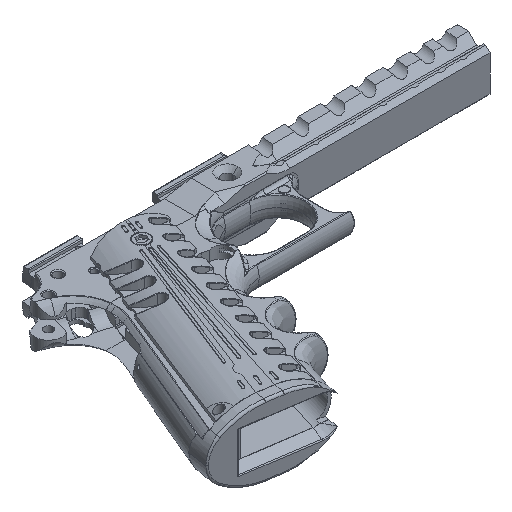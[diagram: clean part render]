
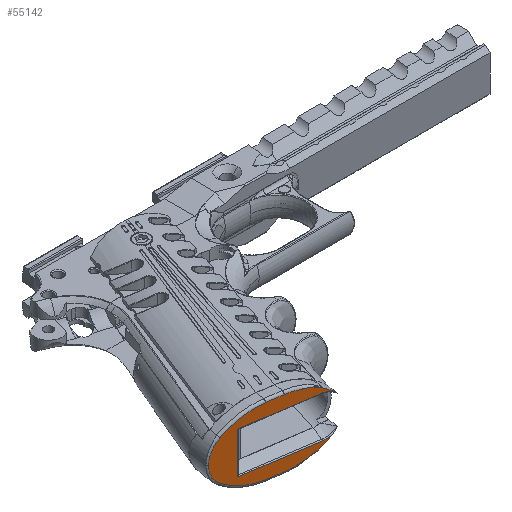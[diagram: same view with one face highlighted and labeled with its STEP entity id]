
A CAD part, isometric view. The second image highlights one B-rep face of the part: STEP entity #55142.
In plain terms, the highlighted face is planar.
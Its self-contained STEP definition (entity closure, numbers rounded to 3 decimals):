
#740 = VERTEX_POINT ( 'NONE', #28184 ) ;
#1054 = VERTEX_POINT ( 'NONE', #53536 ) ;
#1213 = CARTESIAN_POINT ( 'NONE',  ( -13.838, -5.164, 15.002 ) ) ;
#1341 = DIRECTION ( 'NONE',  ( -0.968, 0.25, 0. ) ) ;
#1467 = VERTEX_POINT ( 'NONE', #28141 ) ;
#1565 = DIRECTION ( 'NONE',  ( -0.25, -0.968, 0. ) ) ;
#2685 = AXIS2_PLACEMENT_3D ( 'NONE', #48530, #22746, #52839 ) ;
#5415 = CARTESIAN_POINT ( 'NONE',  ( -35.601, 0.464, -9.336 ) ) ;
#5814 = EDGE_CURVE ( 'NONE', #740, #1467, #17793, .T. ) ;
#6906 = DIRECTION ( 'NONE',  ( -0.25, -0.968, 0. ) ) ;
#7460 = ORIENTED_EDGE ( 'NONE', *, *, #9347, .T. ) ;
#7547 = VERTEX_POINT ( 'NONE', #1213 ) ;
#7964 = CARTESIAN_POINT ( 'NONE',  ( -35.601, 0.464, -9.336 ) ) ;
#8455 = CARTESIAN_POINT ( 'NONE',  ( -21.042, -3.301, -10.872 ) ) ;
#8706 = CARTESIAN_POINT ( 'NONE',  ( -3.333, -7.881, -9.336 ) ) ;
#8812 = CARTESIAN_POINT ( 'NONE',  ( -35.601, 0.464, 0.172 ) ) ;
#8847 = EDGE_LOOP ( 'NONE', ( #16070, #20931, #49724, #31123, #29379, #7460, #43959, #24460, #55542, #18358, #27515, #50691, #26341, #55709, #39166 ) ) ;
#9347 = EDGE_CURVE ( 'NONE', #20665, #36911, #39909, .T. ) ;
#10375 = CARTESIAN_POINT ( 'NONE',  ( -2.664, -8.054, 0. ) ) ;
#10901 = AXIS2_PLACEMENT_3D ( 'NONE', #10375, #40502, #14670 ) ;
#10931 = VERTEX_POINT ( 'NONE', #7964 ) ;
#11095 = CIRCLE ( 'NONE', #32294, 25.874 ) ;
#11402 = EDGE_CURVE ( 'NONE', #1467, #31422, #40404, .T. ) ;
#12796 = DIRECTION ( 'NONE',  ( -0.968, 0.25, 0. ) ) ;
#13134 = EDGE_CURVE ( 'NONE', #34300, #25150, #17911, .T. ) ;
#13143 = DIRECTION ( 'NONE',  ( -0.968, 0.25, 0. ) ) ;
#14338 = CARTESIAN_POINT ( 'NONE',  ( -35.601, 0.464, -0.197 ) ) ;
#14342 = CARTESIAN_POINT ( 'NONE',  ( -26.452, -1.902, -14.417 ) ) ;
#14670 = DIRECTION ( 'NONE',  ( -0.968, 0.25, 0. ) ) ;
#14762 = AXIS2_PLACEMENT_3D ( 'NONE', #15508, #45599, #19800 ) ;
#15508 = CARTESIAN_POINT ( 'NONE',  ( -21.042, -3.301, 10.846 ) ) ;
#15869 = DIRECTION ( 'NONE',  ( 0.968, -0.25, 0. ) ) ;
#16070 = ORIENTED_EDGE ( 'NONE', *, *, #27260, .T. ) ;
#16333 = VERTEX_POINT ( 'NONE', #14342 ) ;
#17274 = LINE ( 'NONE', #41780, #50258 ) ;
#17624 = CIRCLE ( 'NONE', #2685, 24.846 ) ;
#17793 = CIRCLE ( 'NONE', #21756, 9.508 ) ;
#17911 = LINE ( 'NONE', #28651, #39541 ) ;
#18358 = ORIENTED_EDGE ( 'NONE', *, *, #30033, .T. ) ;
#18611 = EDGE_CURVE ( 'NONE', #52695, #1054, #11095, .T. ) ;
#18633 = DIRECTION ( 'NONE',  ( -0.968, 0.25, 0. ) ) ;
#18714 = CARTESIAN_POINT ( 'NONE',  ( 3.48, -9.643, -8.85 ) ) ;
#18730 = CIRCLE ( 'NONE', #35999, 24.846 ) ;
#18989 = VECTOR ( 'NONE', #1341, 1000. ) ;
#19800 = DIRECTION ( 'NONE',  ( -0.968, 0.25, 0. ) ) ;
#20319 = LINE ( 'NONE', #5415, #18989 ) ;
#20665 = VERTEX_POINT ( 'NONE', #47345 ) ;
#20699 = PLANE ( 'NONE',  #49646 ) ;
#20931 = ORIENTED_EDGE ( 'NONE', *, *, #32520, .T. ) ;
#21369 = DIRECTION ( 'NONE',  ( -0.968, 0.25, 0. ) ) ;
#21553 = CARTESIAN_POINT ( 'NONE',  ( -3.616, -7.808, 9.311 ) ) ;
#21756 = AXIS2_PLACEMENT_3D ( 'NONE', #14338, #44456, #18633 ) ;
#22746 = DIRECTION ( 'NONE',  ( -0.25, -0.968, 0. ) ) ;
#24460 = ORIENTED_EDGE ( 'NONE', *, *, #32260, .T. ) ;
#24866 = DIRECTION ( 'NONE',  ( -0.25, -0.968, 0. ) ) ;
#25075 = CARTESIAN_POINT ( 'NONE',  ( -23.833, -2.579, -10.307 ) ) ;
#25150 = VERTEX_POINT ( 'NONE', #34819 ) ;
#25222 = DIRECTION ( 'NONE',  ( -0.968, 0.25, 0. ) ) ;
#25497 = CARTESIAN_POINT ( 'NONE',  ( -14.534, -4.984, 15.002 ) ) ;
#25762 = EDGE_CURVE ( 'NONE', #53487, #20665, #45280, .T. ) ;
#25859 = DIRECTION ( 'NONE',  ( 0.968, -0.25, 0. ) ) ;
#26341 = ORIENTED_EDGE ( 'NONE', *, *, #50733, .T. ) ;
#27244 = CARTESIAN_POINT ( 'NONE',  ( -2.664, -8.054, -0.025 ) ) ;
#27260 = EDGE_CURVE ( 'NONE', #34244, #16333, #17624, .T. ) ;
#27515 = ORIENTED_EDGE ( 'NONE', *, *, #5814, .T. ) ;
#27705 = AXIS2_PLACEMENT_3D ( 'NONE', #27244, #1565, #31617 ) ;
#28141 = CARTESIAN_POINT ( 'NONE',  ( -35.601, 0.464, 9.311 ) ) ;
#28184 = CARTESIAN_POINT ( 'NONE',  ( -39.832, 1.558, 8.247 ) ) ;
#28651 = CARTESIAN_POINT ( 'NONE',  ( -14.534, -4.984, -15.027 ) ) ;
#29379 = ORIENTED_EDGE ( 'NONE', *, *, #25762, .T. ) ;
#29443 = DIRECTION ( 'NONE',  ( 0.968, -0.25, 0. ) ) ;
#30033 = EDGE_CURVE ( 'NONE', #1054, #740, #18730, .T. ) ;
#30694 = CIRCLE ( 'NONE', #14762, 25.874 ) ;
#31123 = ORIENTED_EDGE ( 'NONE', *, *, #46734, .T. ) ;
#31409 = LINE ( 'NONE', #25497, #38819 ) ;
#31422 = VERTEX_POINT ( 'NONE', #47981 ) ;
#31617 = DIRECTION ( 'NONE',  ( -0.968, 0.25, 0. ) ) ;
#32260 = EDGE_CURVE ( 'NONE', #7547, #52695, #31409, .T. ) ;
#32294 = AXIS2_PLACEMENT_3D ( 'NONE', #8455, #38609, #12796 ) ;
#32520 = EDGE_CURVE ( 'NONE', #16333, #34300, #30694, .T. ) ;
#32710 = CARTESIAN_POINT ( 'NONE',  ( -14.534, -4.984, 16.039 ) ) ;
#34244 = VERTEX_POINT ( 'NONE', #53282 ) ;
#34300 = VERTEX_POINT ( 'NONE', #51211 ) ;
#34819 = CARTESIAN_POINT ( 'NONE',  ( -13.838, -5.164, -15.027 ) ) ;
#35051 = EDGE_CURVE ( 'NONE', #39583, #10931, #20319, .T. ) ;
#35999 = AXIS2_PLACEMENT_3D ( 'NONE', #25075, #55162, #29443 ) ;
#36624 = AXIS2_PLACEMENT_3D ( 'NONE', #8812, #38960, #13143 ) ;
#36911 = VERTEX_POINT ( 'NONE', #51225 ) ;
#37058 = DIRECTION ( 'NONE',  ( -0.968, 0.25, 0. ) ) ;
#38108 = CARTESIAN_POINT ( 'NONE',  ( -14.534, -4.984, 16.039 ) ) ;
#38609 = DIRECTION ( 'NONE',  ( -0.25, -0.968, 0. ) ) ;
#38819 = VECTOR ( 'NONE', #21369, 1000. ) ;
#38960 = DIRECTION ( 'NONE',  ( 0.25, 0.968, 0. ) ) ;
#39166 = ORIENTED_EDGE ( 'NONE', *, *, #51722, .T. ) ;
#39541 = VECTOR ( 'NONE', #15869, 1000. ) ;
#39583 = VERTEX_POINT ( 'NONE', #8706 ) ;
#39909 = CIRCLE ( 'NONE', #27705, 10.89 ) ;
#40404 = LINE ( 'NONE', #21553, #51767 ) ;
#40502 = DIRECTION ( 'NONE',  ( -0.25, -0.968, 0. ) ) ;
#41120 = AXIS2_PLACEMENT_3D ( 'NONE', #50655, #24866, #54961 ) ;
#41780 = CARTESIAN_POINT ( 'NONE',  ( -3.333, -7.881, -8.998 ) ) ;
#41970 = DIRECTION ( 'NONE',  ( 0., 0., -1. ) ) ;
#43798 = CIRCLE ( 'NONE', #41120, 31.075 ) ;
#43959 = ORIENTED_EDGE ( 'NONE', *, *, #48716, .T. ) ;
#44456 = DIRECTION ( 'NONE',  ( 0.25, 0.968, 0. ) ) ;
#45280 = CIRCLE ( 'NONE', #10901, 10.89 ) ;
#45288 = CIRCLE ( 'NONE', #46774, 31.075 ) ;
#45479 = CIRCLE ( 'NONE', #36624, 9.508 ) ;
#45599 = DIRECTION ( 'NONE',  ( -0.25, -0.968, 0. ) ) ;
#46734 = EDGE_CURVE ( 'NONE', #25150, #53487, #45288, .T. ) ;
#46774 = AXIS2_PLACEMENT_3D ( 'NONE', #32710, #6906, #37058 ) ;
#47345 = CARTESIAN_POINT ( 'NONE',  ( 7.879, -10.78, -0.012 ) ) ;
#47598 = CARTESIAN_POINT ( 'NONE',  ( -21.042, -3.301, 15.002 ) ) ;
#47981 = CARTESIAN_POINT ( 'NONE',  ( -3.333, -7.881, 9.311 ) ) ;
#48530 = CARTESIAN_POINT ( 'NONE',  ( -23.833, -2.579, 10.282 ) ) ;
#48716 = EDGE_CURVE ( 'NONE', #36911, #7547, #43798, .T. ) ;
#49646 = AXIS2_PLACEMENT_3D ( 'NONE', #38108, #51002, #25222 ) ;
#49724 = ORIENTED_EDGE ( 'NONE', *, *, #13134, .T. ) ;
#50258 = VECTOR ( 'NONE', #41970, 1000. ) ;
#50655 = CARTESIAN_POINT ( 'NONE',  ( -14.534, -4.984, -16.064 ) ) ;
#50691 = ORIENTED_EDGE ( 'NONE', *, *, #11402, .T. ) ;
#50733 = EDGE_CURVE ( 'NONE', #31422, #39583, #17274, .T. ) ;
#51002 = DIRECTION ( 'NONE',  ( 0.25, 0.968, 0. ) ) ;
#51211 = CARTESIAN_POINT ( 'NONE',  ( -21.042, -3.301, -15.027 ) ) ;
#51225 = CARTESIAN_POINT ( 'NONE',  ( 3.48, -9.643, 8.825 ) ) ;
#51722 = EDGE_CURVE ( 'NONE', #10931, #34244, #45479, .T. ) ;
#51767 = VECTOR ( 'NONE', #25859, 1000. ) ;
#52653 = FACE_OUTER_BOUND ( 'NONE', #8847, .T. ) ;
#52695 = VERTEX_POINT ( 'NONE', #47598 ) ;
#52839 = DIRECTION ( 'NONE',  ( -0.968, 0.25, 0. ) ) ;
#53282 = CARTESIAN_POINT ( 'NONE',  ( -39.832, 1.558, -8.272 ) ) ;
#53487 = VERTEX_POINT ( 'NONE', #18714 ) ;
#53536 = CARTESIAN_POINT ( 'NONE',  ( -26.452, -1.902, 14.391 ) ) ;
#54961 = DIRECTION ( 'NONE',  ( -0.968, 0.25, 0. ) ) ;
#55142 = ADVANCED_FACE ( 'NONE', ( #52653 ), #20699, .F. ) ;
#55162 = DIRECTION ( 'NONE',  ( -0.25, -0.968, 0. ) ) ;
#55542 = ORIENTED_EDGE ( 'NONE', *, *, #18611, .T. ) ;
#55709 = ORIENTED_EDGE ( 'NONE', *, *, #35051, .T. ) ;
